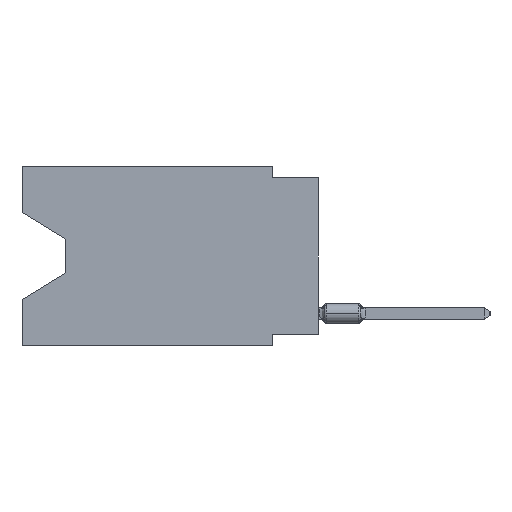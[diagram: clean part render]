
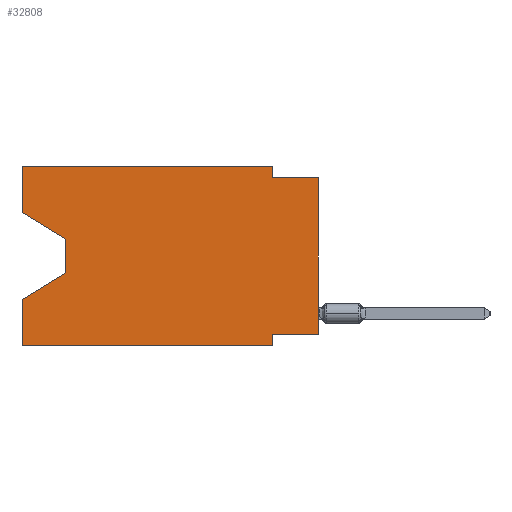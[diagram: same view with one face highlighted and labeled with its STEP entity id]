
A CAD part, left-side view. The second image highlights one B-rep face of the part: STEP entity #32808.
In plain terms, the highlighted planar face has unit normal (-1, 0, 0).
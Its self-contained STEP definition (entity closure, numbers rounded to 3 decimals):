
#40 = CARTESIAN_POINT ( 'NONE',  ( 0., 13.97, -5.893 ) ) ;
#309 = CARTESIAN_POINT ( 'NONE',  ( 0., 13.97, -4.013 ) ) ;
#552 = ORIENTED_EDGE ( 'NONE', *, *, #20852, .F. ) ;
#591 = VERTEX_POINT ( 'NONE', #9811 ) ;
#1320 = CARTESIAN_POINT ( 'NONE',  ( 0., 13.97, -5.893 ) ) ;
#2224 = CARTESIAN_POINT ( 'NONE',  ( 0., 16.383, -2.546 ) ) ;
#3119 = VECTOR ( 'NONE', #32626, 1000. ) ;
#3298 = DIRECTION ( 'NONE',  ( 0., -1., 0. ) ) ;
#4076 = VERTEX_POINT ( 'NONE', #47033 ) ;
#5806 = VECTOR ( 'NONE', #41042, 1000. ) ;
#5861 = LINE ( 'NONE', #2224, #5806 ) ;
#6295 = VERTEX_POINT ( 'NONE', #49388 ) ;
#6434 = AXIS2_PLACEMENT_3D ( 'NONE', #16054, #23836, #40107 ) ;
#6544 = VERTEX_POINT ( 'NONE', #39156 ) ;
#7188 = CARTESIAN_POINT ( 'NONE',  ( 0., 16.383, -9.906 ) ) ;
#7218 = ORIENTED_EDGE ( 'NONE', *, *, #43721, .F. ) ;
#7393 = CARTESIAN_POINT ( 'NONE',  ( 0., 0., -9.271 ) ) ;
#8904 = DIRECTION ( 'NONE',  ( 0., 0., 1. ) ) ;
#9031 = EDGE_CURVE ( 'NONE', #44029, #28872, #43283, .T. ) ;
#9171 = VECTOR ( 'NONE', #12263, 1000. ) ;
#9811 = CARTESIAN_POINT ( 'NONE',  ( 0., 2.54, 0. ) ) ;
#9869 = ORIENTED_EDGE ( 'NONE', *, *, #16322, .T. ) ;
#11951 = DIRECTION ( 'NONE',  ( 0., 0.855, -0.519 ) ) ;
#12263 = DIRECTION ( 'NONE',  ( 0., 0., 1. ) ) ;
#13079 = DIRECTION ( 'NONE',  ( 0., -1., 0. ) ) ;
#13661 = CARTESIAN_POINT ( 'NONE',  ( 0., 2.54, -9.906 ) ) ;
#13724 = LINE ( 'NONE', #29517, #3119 ) ;
#13919 = DIRECTION ( 'NONE',  ( 0., 0., -1. ) ) ;
#15021 = ORIENTED_EDGE ( 'NONE', *, *, #9031, .T. ) ;
#15799 = VECTOR ( 'NONE', #38383, 1000. ) ;
#15903 = LINE ( 'NONE', #31697, #9171 ) ;
#16054 = CARTESIAN_POINT ( 'NONE',  ( 0., 16.383, 0. ) ) ;
#16204 = EDGE_CURVE ( 'NONE', #44979, #4076, #44151, .T. ) ;
#16322 = EDGE_CURVE ( 'NONE', #6544, #44029, #5861, .T. ) ;
#16976 = CARTESIAN_POINT ( 'NONE',  ( 0., 16.383, 0. ) ) ;
#17489 = LINE ( 'NONE', #49057, #34917 ) ;
#18917 = VECTOR ( 'NONE', #11951, 1000. ) ;
#20852 = EDGE_CURVE ( 'NONE', #6295, #591, #48009, .T. ) ;
#21439 = LINE ( 'NONE', #13661, #24156 ) ;
#23836 = DIRECTION ( 'NONE',  ( 1., 0., 0. ) ) ;
#24156 = VECTOR ( 'NONE', #37224, 1000. ) ;
#24435 = VECTOR ( 'NONE', #13079, 1000. ) ;
#26377 = CARTESIAN_POINT ( 'NONE',  ( 0., 0., -9.271 ) ) ;
#26409 = ORIENTED_EDGE ( 'NONE', *, *, #16204, .F. ) ;
#27024 = VERTEX_POINT ( 'NONE', #7393 ) ;
#27348 = EDGE_CURVE ( 'NONE', #30640, #30171, #50371, .T. ) ;
#27607 = ORIENTED_EDGE ( 'NONE', *, *, #44855, .F. ) ;
#27666 = EDGE_CURVE ( 'NONE', #591, #44979, #17489, .T. ) ;
#27692 = EDGE_CURVE ( 'NONE', #40530, #30171, #21439, .T. ) ;
#27960 = PLANE ( 'NONE',  #6434 ) ;
#28872 = VERTEX_POINT ( 'NONE', #1320 ) ;
#28879 = CARTESIAN_POINT ( 'NONE',  ( 0., 16.383, -9.906 ) ) ;
#29517 = CARTESIAN_POINT ( 'NONE',  ( 0., 16.383, 0. ) ) ;
#29942 = VECTOR ( 'NONE', #42122, 1000. ) ;
#30084 = ORIENTED_EDGE ( 'NONE', *, *, #43541, .T. ) ;
#30171 = VERTEX_POINT ( 'NONE', #46361 ) ;
#30224 = ORIENTED_EDGE ( 'NONE', *, *, #27348, .T. ) ;
#30386 = ORIENTED_EDGE ( 'NONE', *, *, #27666, .F. ) ;
#30640 = VERTEX_POINT ( 'NONE', #28879 ) ;
#31697 = CARTESIAN_POINT ( 'NONE',  ( 0., 0., 0. ) ) ;
#32556 = CARTESIAN_POINT ( 'NONE',  ( 0., 16.383, -7.36 ) ) ;
#32626 = DIRECTION ( 'NONE',  ( 0., 0., 1. ) ) ;
#32765 = DIRECTION ( 'NONE',  ( 0., -1., 0. ) ) ;
#32808 = ADVANCED_FACE ( 'NONE', ( #35482 ), #27960, .F. ) ;
#32965 = CARTESIAN_POINT ( 'NONE',  ( 0., 16.383, 0. ) ) ;
#34220 = EDGE_CURVE ( 'NONE', #28872, #49771, #35516, .T. ) ;
#34472 = CARTESIAN_POINT ( 'NONE',  ( 0., 2.54, -0.635 ) ) ;
#34917 = VECTOR ( 'NONE', #13919, 1000. ) ;
#35482 = FACE_OUTER_BOUND ( 'NONE', #45085, .T. ) ;
#35516 = LINE ( 'NONE', #40, #18917 ) ;
#36186 = ORIENTED_EDGE ( 'NONE', *, *, #34220, .T. ) ;
#36351 = VECTOR ( 'NONE', #32765, 1000. ) ;
#37224 = DIRECTION ( 'NONE',  ( 0., 0., -1. ) ) ;
#38383 = DIRECTION ( 'NONE',  ( 0., 0., -1. ) ) ;
#39156 = CARTESIAN_POINT ( 'NONE',  ( 0., 16.383, -2.546 ) ) ;
#40107 = DIRECTION ( 'NONE',  ( 0., 0., -1. ) ) ;
#40530 = VERTEX_POINT ( 'NONE', #49712 ) ;
#40735 = LINE ( 'NONE', #32965, #42209 ) ;
#41042 = DIRECTION ( 'NONE',  ( 0., -0.855, -0.519 ) ) ;
#41273 = EDGE_CURVE ( 'NONE', #30640, #49771, #13724, .T. ) ;
#42122 = DIRECTION ( 'NONE',  ( 0., 1., 0. ) ) ;
#42209 = VECTOR ( 'NONE', #8904, 1000. ) ;
#42650 = LINE ( 'NONE', #26377, #29942 ) ;
#43138 = VECTOR ( 'NONE', #3298, 1000. ) ;
#43283 = LINE ( 'NONE', #46653, #15799 ) ;
#43541 = EDGE_CURVE ( 'NONE', #27024, #4076, #15903, .T. ) ;
#43721 = EDGE_CURVE ( 'NONE', #6544, #6295, #40735, .T. ) ;
#44029 = VERTEX_POINT ( 'NONE', #309 ) ;
#44151 = LINE ( 'NONE', #48286, #36351 ) ;
#44736 = ORIENTED_EDGE ( 'NONE', *, *, #41273, .F. ) ;
#44855 = EDGE_CURVE ( 'NONE', #27024, #40530, #42650, .T. ) ;
#44979 = VERTEX_POINT ( 'NONE', #34472 ) ;
#45085 = EDGE_LOOP ( 'NONE', ( #9869, #15021, #36186, #44736, #30224, #49186, #27607, #30084, #26409, #30386, #552, #7218 ) ) ;
#46361 = CARTESIAN_POINT ( 'NONE',  ( 0., 2.54, -9.906 ) ) ;
#46653 = CARTESIAN_POINT ( 'NONE',  ( 0., 13.97, -4.013 ) ) ;
#47033 = CARTESIAN_POINT ( 'NONE',  ( 0., 0., -0.635 ) ) ;
#48009 = LINE ( 'NONE', #16976, #24435 ) ;
#48286 = CARTESIAN_POINT ( 'NONE',  ( 0., 0., -0.635 ) ) ;
#49057 = CARTESIAN_POINT ( 'NONE',  ( 0., 2.54, 0. ) ) ;
#49186 = ORIENTED_EDGE ( 'NONE', *, *, #27692, .F. ) ;
#49388 = CARTESIAN_POINT ( 'NONE',  ( 0., 16.383, 0. ) ) ;
#49712 = CARTESIAN_POINT ( 'NONE',  ( 0., 2.54, -9.271 ) ) ;
#49771 = VERTEX_POINT ( 'NONE', #32556 ) ;
#50371 = LINE ( 'NONE', #7188, #43138 ) ;
